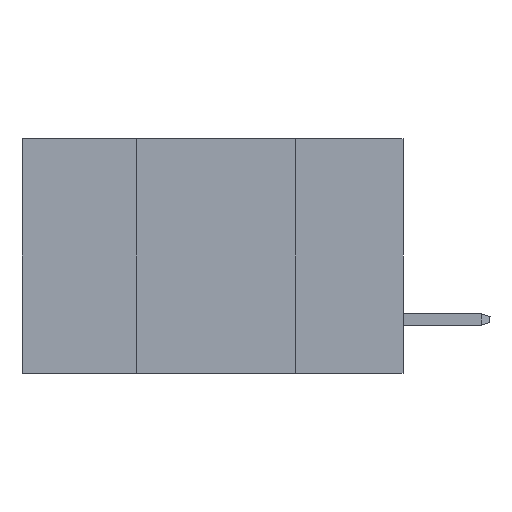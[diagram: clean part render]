
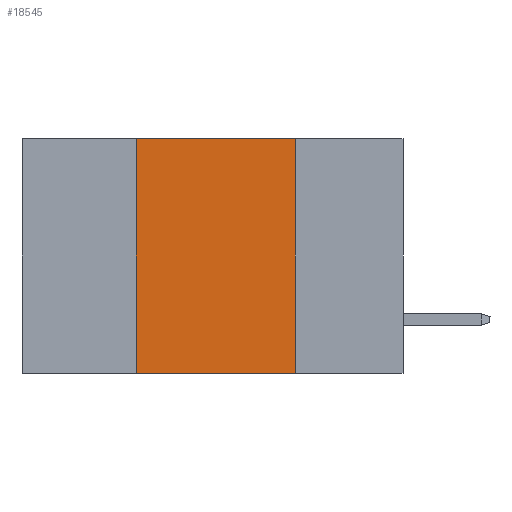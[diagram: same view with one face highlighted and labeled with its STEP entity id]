
A CAD part, left-side view. The second image highlights one B-rep face of the part: STEP entity #18545.
In plain terms, the highlighted planar face has unit normal (-1, 0, 0).
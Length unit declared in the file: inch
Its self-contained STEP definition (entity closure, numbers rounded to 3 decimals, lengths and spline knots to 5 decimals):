
#568 = DIRECTION ( 'NONE',  ( 0., 0., -1. ) ) ;
#1144 = ORIENTED_EDGE ( 'NONE', *, *, #15702, .F. ) ;
#1803 = VECTOR ( 'NONE', #15339, 39.37008 ) ;
#3015 = PLANE ( 'NONE',  #24409 ) ;
#3495 = EDGE_CURVE ( 'NONE', #8193, #28672, #27413, .T. ) ;
#4136 = DIRECTION ( 'NONE',  ( 0., -1., 0. ) ) ;
#5116 = CARTESIAN_POINT ( 'NONE',  ( 0., 0.42, 0. ) ) ;
#5294 = LINE ( 'NONE', #18643, #1803 ) ;
#6300 = CARTESIAN_POINT ( 'NONE',  ( 0., 0.42, 0. ) ) ;
#6766 = DIRECTION ( 'NONE',  ( 1., 0., 0. ) ) ;
#8193 = VERTEX_POINT ( 'NONE', #8330 ) ;
#8330 = CARTESIAN_POINT ( 'NONE',  ( 0., 0.42, -0.37 ) ) ;
#9101 = EDGE_CURVE ( 'NONE', #8193, #9463, #5294, .T. ) ;
#9463 = VERTEX_POINT ( 'NONE', #23773 ) ;
#13799 = VECTOR ( 'NONE', #4136, 39.37008 ) ;
#15326 = LINE ( 'NONE', #26059, #19429 ) ;
#15339 = DIRECTION ( 'NONE',  ( 0., -1., 0. ) ) ;
#15677 = DIRECTION ( 'NONE',  ( 0., 0., -1. ) ) ;
#15702 = EDGE_CURVE ( 'NONE', #28643, #9463, #15326, .T. ) ;
#16146 = CARTESIAN_POINT ( 'NONE',  ( 0., 0.6, 0. ) ) ;
#17695 = EDGE_LOOP ( 'NONE', ( #1144, #26238, #26765, #32253 ) ) ;
#18545 = ADVANCED_FACE ( 'NONE', ( #22343 ), #3015, .F. ) ;
#18643 = CARTESIAN_POINT ( 'NONE',  ( 0., 0.6, -0.37 ) ) ;
#19429 = VECTOR ( 'NONE', #15677, 39.37008 ) ;
#19575 = LINE ( 'NONE', #16146, #13799 ) ;
#20860 = CARTESIAN_POINT ( 'NONE',  ( 0., 0.17, 0. ) ) ;
#22343 = FACE_OUTER_BOUND ( 'NONE', #17695, .T. ) ;
#22385 = DIRECTION ( 'NONE',  ( 0., 0., 1. ) ) ;
#23773 = CARTESIAN_POINT ( 'NONE',  ( 0., 0.17, -0.37 ) ) ;
#24409 = AXIS2_PLACEMENT_3D ( 'NONE', #27710, #6766, #568 ) ;
#26059 = CARTESIAN_POINT ( 'NONE',  ( 0., 0.17, 0. ) ) ;
#26238 = ORIENTED_EDGE ( 'NONE', *, *, #33188, .F. ) ;
#26378 = VECTOR ( 'NONE', #22385, 39.37008 ) ;
#26765 = ORIENTED_EDGE ( 'NONE', *, *, #3495, .F. ) ;
#27413 = LINE ( 'NONE', #6300, #26378 ) ;
#27710 = CARTESIAN_POINT ( 'NONE',  ( 0., 0.6, 0. ) ) ;
#28643 = VERTEX_POINT ( 'NONE', #20860 ) ;
#28672 = VERTEX_POINT ( 'NONE', #5116 ) ;
#32253 = ORIENTED_EDGE ( 'NONE', *, *, #9101, .T. ) ;
#33188 = EDGE_CURVE ( 'NONE', #28672, #28643, #19575, .T. ) ;
